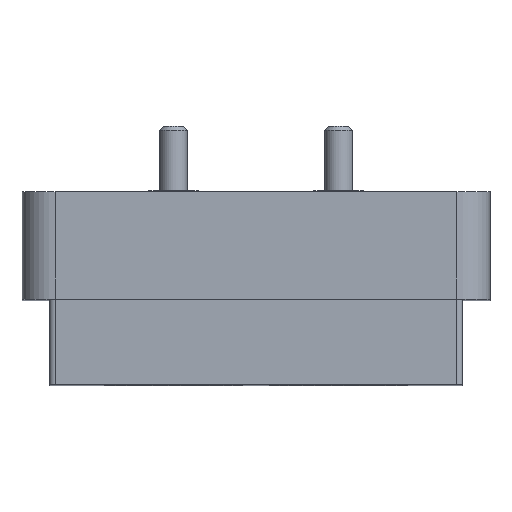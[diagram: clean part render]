
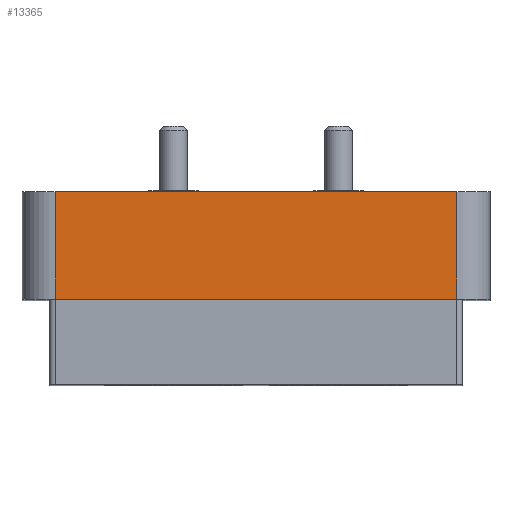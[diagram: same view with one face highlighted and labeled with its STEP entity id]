
A CAD part, top view. The second image highlights one B-rep face of the part: STEP entity #13365.
In plain terms, the highlighted planar face has unit normal (0, 0, 1).
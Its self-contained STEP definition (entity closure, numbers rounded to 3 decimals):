
#31 = EDGE_LOOP ( 'NONE', ( #12892, #5385, #7891, #8914 ) ) ;
#118 = LINE ( 'NONE', #12953, #15283 ) ;
#416 = EDGE_CURVE ( 'NONE', #3476, #14047, #2551, .T. ) ;
#849 = CARTESIAN_POINT ( 'NONE',  ( 7.3, 2.1, 16. ) ) ;
#941 = VERTEX_POINT ( 'NONE', #3578 ) ;
#972 = VECTOR ( 'NONE', #11965, 1000. ) ;
#1744 = LINE ( 'NONE', #12375, #2994 ) ;
#1747 = CARTESIAN_POINT ( 'NONE',  ( 0., 3.55, 16. ) ) ;
#2551 = LINE ( 'NONE', #7225, #972 ) ;
#2994 = VECTOR ( 'NONE', #7718, 1000. ) ;
#3476 = VERTEX_POINT ( 'NONE', #4011 ) ;
#3578 = CARTESIAN_POINT ( 'NONE',  ( 7.3, 6., 16. ) ) ;
#4011 = CARTESIAN_POINT ( 'NONE',  ( -7.3, 2.1, 16. ) ) ;
#4025 = CARTESIAN_POINT ( 'NONE',  ( -7.3, 5., 16. ) ) ;
#5169 = EDGE_CURVE ( 'NONE', #6756, #941, #118, .T. ) ;
#5385 = ORIENTED_EDGE ( 'NONE', *, *, #5169, .F. ) ;
#5942 = AXIS2_PLACEMENT_3D ( 'NONE', #1747, #8417, #13158 ) ;
#6217 = CARTESIAN_POINT ( 'NONE',  ( -7.3, 6., 16. ) ) ;
#6234 = FACE_OUTER_BOUND ( 'NONE', #31, .T. ) ;
#6756 = VERTEX_POINT ( 'NONE', #6217 ) ;
#7225 = CARTESIAN_POINT ( 'NONE',  ( -7.3, 2.1, 16. ) ) ;
#7507 = DIRECTION ( 'NONE',  ( 0., -1., 0. ) ) ;
#7718 = DIRECTION ( 'NONE',  ( 0., 1., 0. ) ) ;
#7747 = LINE ( 'NONE', #4025, #13699 ) ;
#7866 = EDGE_CURVE ( 'NONE', #14047, #941, #1744, .T. ) ;
#7891 = ORIENTED_EDGE ( 'NONE', *, *, #15269, .T. ) ;
#8417 = DIRECTION ( 'NONE',  ( 0., 0., 1. ) ) ;
#8914 = ORIENTED_EDGE ( 'NONE', *, *, #416, .T. ) ;
#11040 = PLANE ( 'NONE',  #5942 ) ;
#11762 = DIRECTION ( 'NONE',  ( 1., 0., 0. ) ) ;
#11965 = DIRECTION ( 'NONE',  ( 1., 0., 0. ) ) ;
#12375 = CARTESIAN_POINT ( 'NONE',  ( 7.3, 2.1, 16. ) ) ;
#12892 = ORIENTED_EDGE ( 'NONE', *, *, #7866, .T. ) ;
#12953 = CARTESIAN_POINT ( 'NONE',  ( 0., 6., 16. ) ) ;
#13158 = DIRECTION ( 'NONE',  ( 1., 0., 0. ) ) ;
#13365 = ADVANCED_FACE ( 'NONE', ( #6234 ), #11040, .T. ) ;
#13699 = VECTOR ( 'NONE', #7507, 1000. ) ;
#14047 = VERTEX_POINT ( 'NONE', #849 ) ;
#15269 = EDGE_CURVE ( 'NONE', #6756, #3476, #7747, .T. ) ;
#15283 = VECTOR ( 'NONE', #11762, 1000. ) ;
